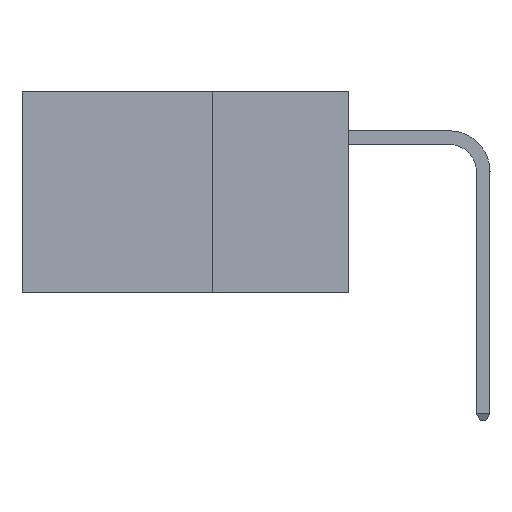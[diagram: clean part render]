
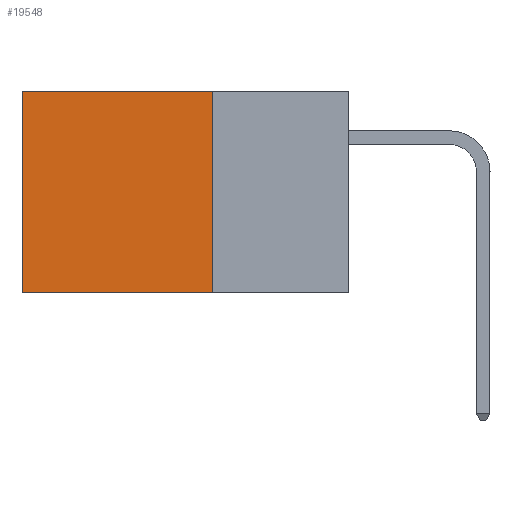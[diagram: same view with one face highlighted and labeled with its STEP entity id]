
A CAD part, left-side view. The second image highlights one B-rep face of the part: STEP entity #19548.
In plain terms, the highlighted planar face has unit normal (-1, 0, 0).
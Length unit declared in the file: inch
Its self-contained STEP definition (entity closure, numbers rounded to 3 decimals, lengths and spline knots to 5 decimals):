
#1468 = LINE ( 'NONE', #8800, #10785 ) ;
#2070 = FACE_OUTER_BOUND ( 'NONE', #20456, .T. ) ;
#2592 = ORIENTED_EDGE ( 'NONE', *, *, #22188, .T. ) ;
#2664 = CARTESIAN_POINT ( 'NONE',  ( 0.2875, 0.25, 0. ) ) ;
#3167 = CARTESIAN_POINT ( 'NONE',  ( 0.2875, 0.6, 0. ) ) ;
#3610 = VERTEX_POINT ( 'NONE', #21658 ) ;
#5084 = VERTEX_POINT ( 'NONE', #7049 ) ;
#5421 = AXIS2_PLACEMENT_3D ( 'NONE', #11996, #6480, #15663 ) ;
#6079 = EDGE_CURVE ( 'NONE', #5084, #7248, #14130, .T. ) ;
#6480 = DIRECTION ( 'NONE',  ( 1., 0., 0. ) ) ;
#7049 = CARTESIAN_POINT ( 'NONE',  ( 0.2875, 0.25, 0. ) ) ;
#7248 = VERTEX_POINT ( 'NONE', #13570 ) ;
#8649 = VECTOR ( 'NONE', #19616, 39.37008 ) ;
#8800 = CARTESIAN_POINT ( 'NONE',  ( 0.2875, 0.25, 0. ) ) ;
#10730 = EDGE_CURVE ( 'NONE', #5084, #10886, #1468, .T. ) ;
#10785 = VECTOR ( 'NONE', #21456, 39.37008 ) ;
#10886 = VERTEX_POINT ( 'NONE', #11040 ) ;
#11040 = CARTESIAN_POINT ( 'NONE',  ( 0.2875, 0.6, 0. ) ) ;
#11483 = ORIENTED_EDGE ( 'NONE', *, *, #16088, .F. ) ;
#11996 = CARTESIAN_POINT ( 'NONE',  ( 0.2875, 0.25, 0. ) ) ;
#12260 = ORIENTED_EDGE ( 'NONE', *, *, #10730, .T. ) ;
#13516 = LINE ( 'NONE', #18729, #17788 ) ;
#13570 = CARTESIAN_POINT ( 'NONE',  ( 0.2875, 0.25, -0.37 ) ) ;
#13821 = PLANE ( 'NONE',  #5421 ) ;
#14130 = LINE ( 'NONE', #2664, #23099 ) ;
#15663 = DIRECTION ( 'NONE',  ( 0., 0., -1. ) ) ;
#16088 = EDGE_CURVE ( 'NONE', #7248, #3610, #13516, .T. ) ;
#16942 = DIRECTION ( 'NONE',  ( 0., 1., 0. ) ) ;
#17788 = VECTOR ( 'NONE', #16942, 39.37008 ) ;
#18729 = CARTESIAN_POINT ( 'NONE',  ( 0.2875, 0.25, -0.37 ) ) ;
#19150 = DIRECTION ( 'NONE',  ( 0., 0., -1. ) ) ;
#19330 = ORIENTED_EDGE ( 'NONE', *, *, #6079, .F. ) ;
#19548 = ADVANCED_FACE ( 'NONE', ( #2070 ), #13821, .F. ) ;
#19616 = DIRECTION ( 'NONE',  ( 0., 0., -1. ) ) ;
#20456 = EDGE_LOOP ( 'NONE', ( #2592, #11483, #19330, #12260 ) ) ;
#21456 = DIRECTION ( 'NONE',  ( 0., 1., 0. ) ) ;
#21658 = CARTESIAN_POINT ( 'NONE',  ( 0.2875, 0.6, -0.37 ) ) ;
#22188 = EDGE_CURVE ( 'NONE', #10886, #3610, #22504, .T. ) ;
#22504 = LINE ( 'NONE', #3167, #8649 ) ;
#23099 = VECTOR ( 'NONE', #19150, 39.37008 ) ;
